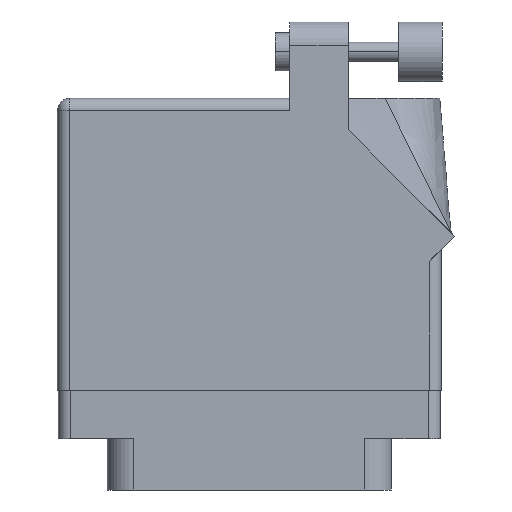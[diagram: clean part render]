
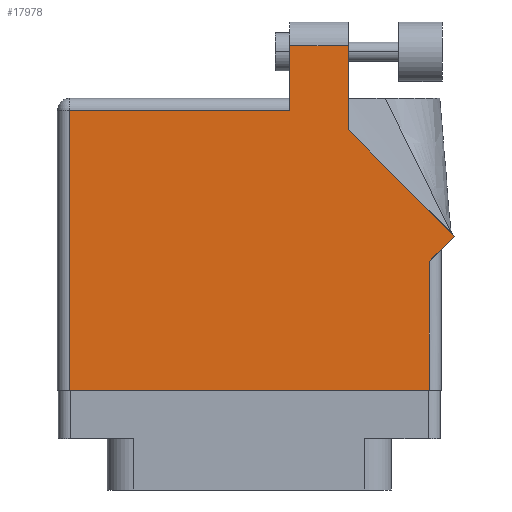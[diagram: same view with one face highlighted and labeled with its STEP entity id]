
A CAD part, front view. The second image highlights one B-rep face of the part: STEP entity #17978.
In plain terms, the highlighted face is planar.
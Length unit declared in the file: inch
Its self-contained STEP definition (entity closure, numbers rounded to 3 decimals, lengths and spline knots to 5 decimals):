
#400 = VECTOR ( 'NONE', #8080, 39.37008 ) ;
#1533 = CARTESIAN_POINT ( 'NONE',  ( 1.07571, 0.70771, 0.455 ) ) ;
#1608 = CARTESIAN_POINT ( 'NONE',  ( -0.943, 1.368, 0.455 ) ) ;
#1889 = VECTOR ( 'NONE', #5725, 39.37008 ) ;
#2014 = VECTOR ( 'NONE', #35504, 39.37008 ) ;
#2240 = VERTEX_POINT ( 'NONE', #17775 ) ;
#3052 = EDGE_CURVE ( 'NONE', #5398, #22109, #35194, .T. ) ;
#3054 = DIRECTION ( 'NONE',  ( 0., 1., 0. ) ) ;
#3288 = VERTEX_POINT ( 'NONE', #1608 ) ;
#3368 = LINE ( 'NONE', #12289, #18661 ) ;
#4520 = VERTEX_POINT ( 'NONE', #8375 ) ;
#4996 = ORIENTED_EDGE ( 'NONE', *, *, #33330, .T. ) ;
#5305 = EDGE_LOOP ( 'NONE', ( #23057, #13310, #31689, #29236, #4996, #14525, #28150, #9188, #28060 ) ) ;
#5398 = VERTEX_POINT ( 'NONE', #32352 ) ;
#5629 = CARTESIAN_POINT ( 'NONE',  ( 0.212, 1.705, 0.455 ) ) ;
#5725 = DIRECTION ( 'NONE',  ( 0.707, 0.707, 0. ) ) ;
#6282 = CARTESIAN_POINT ( 'NONE',  ( 0.943, 0.575, 0.455 ) ) ;
#7473 = CARTESIAN_POINT ( 'NONE',  ( -1.005, -0.1, 0.455 ) ) ;
#8080 = DIRECTION ( 'NONE',  ( -1., 0., 0. ) ) ;
#8375 = CARTESIAN_POINT ( 'NONE',  ( 0.519, 1.26442, 0.455 ) ) ;
#9188 = ORIENTED_EDGE ( 'NONE', *, *, #22907, .T. ) ;
#9285 = LINE ( 'NONE', #14022, #1889 ) ;
#9525 = EDGE_CURVE ( 'NONE', #4520, #16118, #18405, .T. ) ;
#10650 = DIRECTION ( 'NONE',  ( 0., -1., 0. ) ) ;
#10961 = VERTEX_POINT ( 'NONE', #15307 ) ;
#11172 = CARTESIAN_POINT ( 'NONE',  ( -1.005, 1.43, 0.455 ) ) ;
#12208 = VECTOR ( 'NONE', #26245, 39.37008 ) ;
#12289 = CARTESIAN_POINT ( 'NONE',  ( 0.943, 0.637, 0.455 ) ) ;
#12731 = VECTOR ( 'NONE', #24891, 39.37008 ) ;
#13005 = VECTOR ( 'NONE', #24279, 39.37008 ) ;
#13310 = ORIENTED_EDGE ( 'NONE', *, *, #14350, .T. ) ;
#13565 = LINE ( 'NONE', #16573, #19243 ) ;
#13740 = PLANE ( 'NONE',  #14771 ) ;
#14022 = CARTESIAN_POINT ( 'NONE',  ( 1.005, 0.637, 0.455 ) ) ;
#14350 = EDGE_CURVE ( 'NONE', #16118, #2240, #27810, .T. ) ;
#14525 = ORIENTED_EDGE ( 'NONE', *, *, #3052, .T. ) ;
#14771 = AXIS2_PLACEMENT_3D ( 'NONE', #11172, #16901, #33667 ) ;
#15307 = CARTESIAN_POINT ( 'NONE',  ( 1.07571, 0.70771, 0.455 ) ) ;
#16041 = EDGE_CURVE ( 'NONE', #18976, #3288, #24636, .T. ) ;
#16113 = LINE ( 'NONE', #1533, #12208 ) ;
#16118 = VERTEX_POINT ( 'NONE', #35860 ) ;
#16353 = VERTEX_POINT ( 'NONE', #6282 ) ;
#16573 = CARTESIAN_POINT ( 'NONE',  ( 0.212, 1.43, 0.455 ) ) ;
#16901 = DIRECTION ( 'NONE',  ( 0., 0., -1. ) ) ;
#17775 = CARTESIAN_POINT ( 'NONE',  ( 0.212, 1.705, 0.455 ) ) ;
#17978 = ADVANCED_FACE ( 'NONE', ( #24567 ), #13740, .F. ) ;
#18405 = LINE ( 'NONE', #33748, #12731 ) ;
#18661 = VECTOR ( 'NONE', #3054, 39.37008 ) ;
#18976 = VERTEX_POINT ( 'NONE', #32519 ) ;
#19243 = VECTOR ( 'NONE', #35784, 39.37008 ) ;
#19294 = EDGE_CURVE ( 'NONE', #22109, #16353, #3368, .T. ) ;
#22109 = VERTEX_POINT ( 'NONE', #32759 ) ;
#22208 = LINE ( 'NONE', #35594, #23931 ) ;
#22907 = EDGE_CURVE ( 'NONE', #16353, #10961, #9285, .T. ) ;
#23057 = ORIENTED_EDGE ( 'NONE', *, *, #9525, .T. ) ;
#23931 = VECTOR ( 'NONE', #10650, 39.37008 ) ;
#24279 = DIRECTION ( 'NONE',  ( 1., 0., 0. ) ) ;
#24567 = FACE_OUTER_BOUND ( 'NONE', #5305, .T. ) ;
#24636 = LINE ( 'NONE', #30047, #2014 ) ;
#24891 = DIRECTION ( 'NONE',  ( 0., 1., 0. ) ) ;
#26245 = DIRECTION ( 'NONE',  ( -0.707, 0.707, 0. ) ) ;
#27810 = LINE ( 'NONE', #5629, #400 ) ;
#28060 = ORIENTED_EDGE ( 'NONE', *, *, #31456, .T. ) ;
#28150 = ORIENTED_EDGE ( 'NONE', *, *, #19294, .T. ) ;
#29236 = ORIENTED_EDGE ( 'NONE', *, *, #16041, .T. ) ;
#30047 = CARTESIAN_POINT ( 'NONE',  ( -1.005, 1.368, 0.455 ) ) ;
#31456 = EDGE_CURVE ( 'NONE', #10961, #4520, #16113, .T. ) ;
#31689 = ORIENTED_EDGE ( 'NONE', *, *, #32360, .T. ) ;
#32352 = CARTESIAN_POINT ( 'NONE',  ( -0.943, -0.1, 0.455 ) ) ;
#32360 = EDGE_CURVE ( 'NONE', #2240, #18976, #13565, .T. ) ;
#32519 = CARTESIAN_POINT ( 'NONE',  ( 0.212, 1.368, 0.455 ) ) ;
#32759 = CARTESIAN_POINT ( 'NONE',  ( 0.943, -0.1, 0.455 ) ) ;
#33330 = EDGE_CURVE ( 'NONE', #3288, #5398, #22208, .T. ) ;
#33667 = DIRECTION ( 'NONE',  ( -1., 0., 0. ) ) ;
#33748 = CARTESIAN_POINT ( 'NONE',  ( 0.519, 1.26442, 0.455 ) ) ;
#35194 = LINE ( 'NONE', #7473, #13005 ) ;
#35504 = DIRECTION ( 'NONE',  ( -1., 0., 0. ) ) ;
#35594 = CARTESIAN_POINT ( 'NONE',  ( -0.943, -0.1, 0.455 ) ) ;
#35784 = DIRECTION ( 'NONE',  ( 0., -1., 0. ) ) ;
#35860 = CARTESIAN_POINT ( 'NONE',  ( 0.519, 1.705, 0.455 ) ) ;
